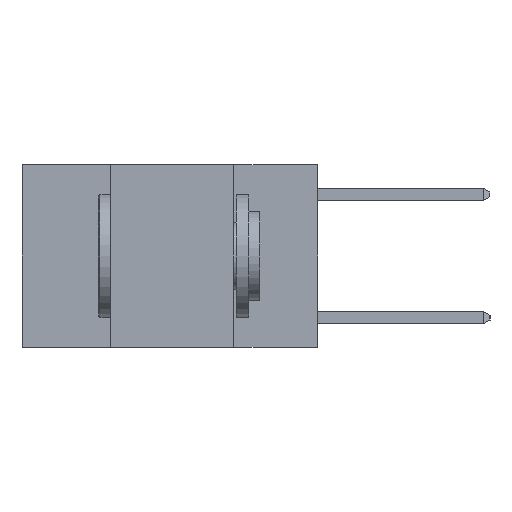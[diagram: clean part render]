
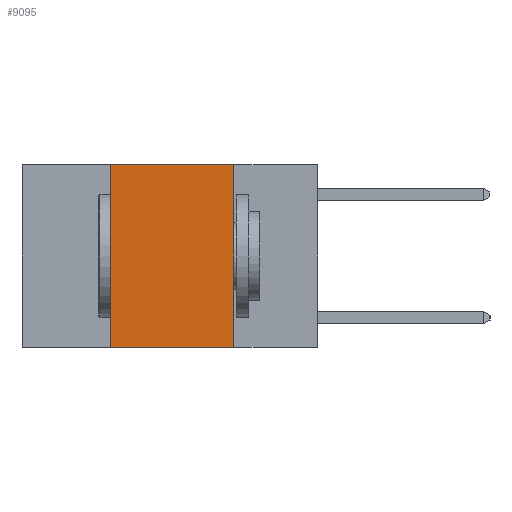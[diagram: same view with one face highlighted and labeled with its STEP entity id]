
A CAD part, left-side view. The second image highlights one B-rep face of the part: STEP entity #9095.
In plain terms, the highlighted planar face has unit normal (-1, 0, 0).
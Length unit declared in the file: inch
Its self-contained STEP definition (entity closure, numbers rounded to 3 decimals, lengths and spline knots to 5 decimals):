
#145 = EDGE_CURVE ( 'NONE', #2901, #5469, #4714, .T. ) ;
#236 = EDGE_LOOP ( 'NONE', ( #1078, #5260, #1535, #8215 ) ) ;
#487 = VERTEX_POINT ( 'NONE', #2238 ) ;
#659 = CARTESIAN_POINT ( 'NONE',  ( 0., 0.17, -0.37 ) ) ;
#751 = LINE ( 'NONE', #4758, #8269 ) ;
#1078 = ORIENTED_EDGE ( 'NONE', *, *, #5971, .F. ) ;
#1167 = VERTEX_POINT ( 'NONE', #659 ) ;
#1535 = ORIENTED_EDGE ( 'NONE', *, *, #145, .F. ) ;
#2122 = LINE ( 'NONE', #5107, #9157 ) ;
#2238 = CARTESIAN_POINT ( 'NONE',  ( 0., 0.17, 0. ) ) ;
#2855 = DIRECTION ( 'NONE',  ( 1., 0., 0. ) ) ;
#2901 = VERTEX_POINT ( 'NONE', #6358 ) ;
#3474 = DIRECTION ( 'NONE',  ( 0., -1., 0. ) ) ;
#3488 = CARTESIAN_POINT ( 'NONE',  ( 0., 0.6, 0. ) ) ;
#4065 = LINE ( 'NONE', #3488, #5852 ) ;
#4714 = LINE ( 'NONE', #5118, #6914 ) ;
#4745 = DIRECTION ( 'NONE',  ( 0., -1., 0. ) ) ;
#4758 = CARTESIAN_POINT ( 'NONE',  ( 0., 0.6, -0.37 ) ) ;
#5045 = PLANE ( 'NONE',  #8790 ) ;
#5096 = DIRECTION ( 'NONE',  ( 0., 0., -1. ) ) ;
#5107 = CARTESIAN_POINT ( 'NONE',  ( 0., 0.17, 0. ) ) ;
#5118 = CARTESIAN_POINT ( 'NONE',  ( 0., 0.42, 0. ) ) ;
#5260 = ORIENTED_EDGE ( 'NONE', *, *, #6378, .F. ) ;
#5469 = VERTEX_POINT ( 'NONE', #7363 ) ;
#5519 = DIRECTION ( 'NONE',  ( 0., 0., 1. ) ) ;
#5852 = VECTOR ( 'NONE', #3474, 39.37008 ) ;
#5971 = EDGE_CURVE ( 'NONE', #487, #1167, #2122, .T. ) ;
#6072 = EDGE_CURVE ( 'NONE', #2901, #1167, #751, .T. ) ;
#6358 = CARTESIAN_POINT ( 'NONE',  ( 0., 0.42, -0.37 ) ) ;
#6378 = EDGE_CURVE ( 'NONE', #5469, #487, #4065, .T. ) ;
#6539 = CARTESIAN_POINT ( 'NONE',  ( 0., 0.6, 0. ) ) ;
#6580 = FACE_OUTER_BOUND ( 'NONE', #236, .T. ) ;
#6914 = VECTOR ( 'NONE', #5519, 39.37008 ) ;
#7363 = CARTESIAN_POINT ( 'NONE',  ( 0., 0.42, 0. ) ) ;
#7934 = DIRECTION ( 'NONE',  ( 0., 0., -1. ) ) ;
#8215 = ORIENTED_EDGE ( 'NONE', *, *, #6072, .T. ) ;
#8269 = VECTOR ( 'NONE', #4745, 39.37008 ) ;
#8790 = AXIS2_PLACEMENT_3D ( 'NONE', #6539, #2855, #7934 ) ;
#9095 = ADVANCED_FACE ( 'NONE', ( #6580 ), #5045, .F. ) ;
#9157 = VECTOR ( 'NONE', #5096, 39.37008 ) ;
